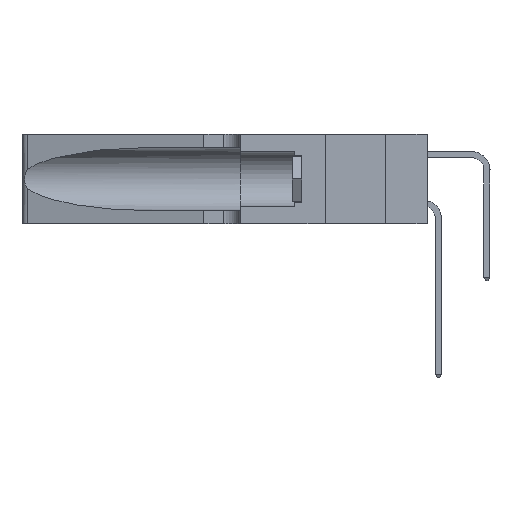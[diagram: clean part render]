
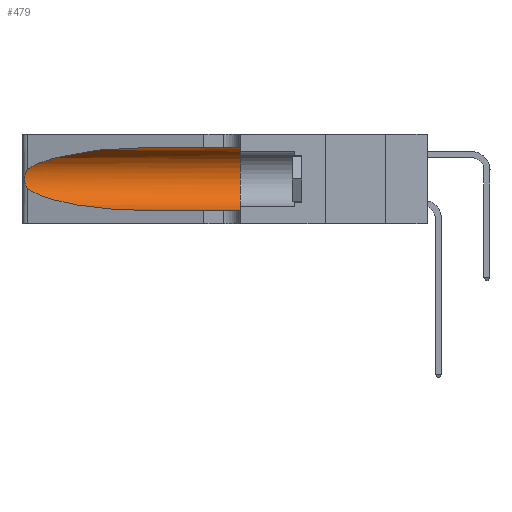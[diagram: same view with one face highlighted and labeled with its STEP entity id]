
A CAD part, left-side view. The second image highlights one B-rep face of the part: STEP entity #479.
In plain terms, the highlighted cylindrical face has radius 3.308 mm (diameter 6.617 mm), a partial arc.
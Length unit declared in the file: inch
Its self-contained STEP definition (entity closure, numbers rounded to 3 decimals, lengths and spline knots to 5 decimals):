
#324 = EDGE_CURVE ( 'NONE', #16394, #5840, #4225, .T. ) ;
#479 = ADVANCED_FACE ( 'NONE', ( #18718 ), #23139, .F. ) ;
#1577 = ORIENTED_EDGE ( 'NONE', *, *, #3728, .T. ) ;
#1714 = CARTESIAN_POINT ( 'NONE',  ( 0.1305, 0.35, 0.31525 ) ) ;
#1887 = CARTESIAN_POINT ( 'NONE',  ( 0.25639, 1.23186, 0.15144 ) ) ;
#2114 = EDGE_LOOP ( 'NONE', ( #1577, #14089, #24258, #11299, #9161, #21161 ) ) ;
#3728 = EDGE_CURVE ( 'NONE', #9143, #12428, #3777, .T. ) ;
#3777 =( BOUNDED_CURVE ( )  B_SPLINE_CURVE ( 3, ( #7094, #5178, #16529, #20314 ),
 .UNSPECIFIED., .F., .T. ) 
 B_SPLINE_CURVE_WITH_KNOTS ( ( 4, 4 ),
 ( 1.5708, 2.84003 ),
 .UNSPECIFIED. ) 
 CURVE ( )  GEOMETRIC_REPRESENTATION_ITEM ( )  RATIONAL_B_SPLINE_CURVE ( ( 1., 0.87, 0.87, 1. ) ) 
 REPRESENTATION_ITEM ( '' )  );
#3819 = CARTESIAN_POINT ( 'NONE',  ( 0.25487, 1.22718, 0.14631 ) ) ;
#4225 =( BOUNDED_CURVE ( )  B_SPLINE_CURVE ( 3, ( #23592, #22608, #22773, #18902 ),
 .UNSPECIFIED., .F., .T. ) 
 B_SPLINE_CURVE_WITH_KNOTS ( ( 4, 4 ),
 ( 3.44316, 4.71239 ),
 .UNSPECIFIED. ) 
 CURVE ( )  GEOMETRIC_REPRESENTATION_ITEM ( )  RATIONAL_B_SPLINE_CURVE ( ( 1., 0.87, 0.87, 1. ) ) 
 REPRESENTATION_ITEM ( '' )  );
#4977 = EDGE_CURVE ( 'NONE', #21585, #9734, #11578, .T. ) ;
#5178 = CARTESIAN_POINT ( 'NONE',  ( 0.18966, 0.96281, 0.31525 ) ) ;
#5443 = LINE ( 'NONE', #18367, #14940 ) ;
#5587 = CARTESIAN_POINT ( 'NONE',  ( 0.25487, 1.22718, 0.22369 ) ) ;
#5673 = CARTESIAN_POINT ( 'NONE',  ( 0.25639, 1.23184, 0.21858 ) ) ;
#5686 = CARTESIAN_POINT ( 'NONE',  ( 0.1305, 0.72297, 0.05475 ) ) ;
#5840 = VERTEX_POINT ( 'NONE', #5686 ) ;
#6756 = CARTESIAN_POINT ( 'NONE',  ( 0.1305, 0.72297, 0.31525 ) ) ;
#7094 = CARTESIAN_POINT ( 'NONE',  ( 0.1305, 0.72297, 0.31525 ) ) ;
#7126 = DIRECTION ( 'NONE',  ( 0., 1., 0. ) ) ;
#7581 = CARTESIAN_POINT ( 'NONE',  ( 0.25854, 1.2359, 0.20912 ) ) ;
#8857 = DIRECTION ( 'NONE',  ( 0., 0., -1. ) ) ;
#8878 = CARTESIAN_POINT ( 'NONE',  ( 0.1305, 0.35, 0.05475 ) ) ;
#9143 = VERTEX_POINT ( 'NONE', #6756 ) ;
#9161 = ORIENTED_EDGE ( 'NONE', *, *, #4977, .F. ) ;
#9429 = CARTESIAN_POINT ( 'NONE',  ( 0.1305, 1.61858, 0.185 ) ) ;
#9481 = CARTESIAN_POINT ( 'NONE',  ( 0.26075, 1.23896, 0.19203 ) ) ;
#9734 = VERTEX_POINT ( 'NONE', #8878 ) ;
#10153 = AXIS2_PLACEMENT_3D ( 'NONE', #9429, #11488, #8857 ) ;
#11299 = ORIENTED_EDGE ( 'NONE', *, *, #22690, .T. ) ;
#11385 = CARTESIAN_POINT ( 'NONE',  ( 0.26017, 1.23833, 0.17102 ) ) ;
#11488 = DIRECTION ( 'NONE',  ( 0., -1., 0. ) ) ;
#11578 = CIRCLE ( 'NONE', #17966, 0.13025 ) ;
#12428 = VERTEX_POINT ( 'NONE', #16102 ) ;
#13272 = CARTESIAN_POINT ( 'NONE',  ( 0.25789, 1.23486, 0.15765 ) ) ;
#13274 = CARTESIAN_POINT ( 'NONE',  ( 0.25487, 1.22718, 0.14631 ) ) ;
#14089 = ORIENTED_EDGE ( 'NONE', *, *, #24045, .T. ) ;
#14370 = LINE ( 'NONE', #21673, #23793 ) ;
#14940 = VECTOR ( 'NONE', #24059, 39.37008 ) ;
#15016 = EDGE_CURVE ( 'NONE', #9143, #21585, #14370, .T. ) ;
#15114 = CARTESIAN_POINT ( 'NONE',  ( 0.25555, 1.22994, 0.2215 ) ) ;
#15202 = CARTESIAN_POINT ( 'NONE',  ( 0.25555, 1.22993, 0.14849 ) ) ;
#16102 = CARTESIAN_POINT ( 'NONE',  ( 0.25487, 1.22718, 0.22369 ) ) ;
#16394 = VERTEX_POINT ( 'NONE', #13274 ) ;
#16529 = CARTESIAN_POINT ( 'NONE',  ( 0.2373, 1.15595, 0.28018 ) ) ;
#17892 = DIRECTION ( 'NONE',  ( 0., -1., 0. ) ) ;
#17966 = AXIS2_PLACEMENT_3D ( 'NONE', #18440, #7126, #20348 ) ;
#18367 = CARTESIAN_POINT ( 'NONE',  ( 0.1305, 1.61858, 0.05475 ) ) ;
#18440 = CARTESIAN_POINT ( 'NONE',  ( 0.1305, 0.35, 0.185 ) ) ;
#18718 = FACE_OUTER_BOUND ( 'NONE', #2114, .T. ) ;
#18900 = CARTESIAN_POINT ( 'NONE',  ( 0.25787, 1.23484, 0.2124 ) ) ;
#18902 = CARTESIAN_POINT ( 'NONE',  ( 0.1305, 0.72297, 0.05475 ) ) ;
#20314 = CARTESIAN_POINT ( 'NONE',  ( 0.25487, 1.22718, 0.22369 ) ) ;
#20348 = DIRECTION ( 'NONE',  ( 0., 0., 1. ) ) ;
#20794 = CARTESIAN_POINT ( 'NONE',  ( 0.26018, 1.23835, 0.19895 ) ) ;
#21161 = ORIENTED_EDGE ( 'NONE', *, *, #15016, .F. ) ;
#21368 = CARTESIAN_POINT ( 'NONE',  ( 0.25856, 1.23593, 0.16098 ) ) ;
#21585 = VERTEX_POINT ( 'NONE', #1714 ) ;
#21673 = CARTESIAN_POINT ( 'NONE',  ( 0.1305, 1.61858, 0.31525 ) ) ;
#22608 = CARTESIAN_POINT ( 'NONE',  ( 0.2373, 1.15595, 0.08982 ) ) ;
#22686 = CARTESIAN_POINT ( 'NONE',  ( 0.26075, 1.23896, 0.178 ) ) ;
#22690 = EDGE_CURVE ( 'NONE', #5840, #9734, #5443, .T. ) ;
#22773 = CARTESIAN_POINT ( 'NONE',  ( 0.18966, 0.96281, 0.05475 ) ) ;
#23139 = CYLINDRICAL_SURFACE ( 'NONE', #10153, 0.13025 ) ;
#23592 = CARTESIAN_POINT ( 'NONE',  ( 0.25487, 1.22718, 0.14631 ) ) ;
#23793 = VECTOR ( 'NONE', #17892, 39.37008 ) ;
#24045 = EDGE_CURVE ( 'NONE', #12428, #16394, #24094, .T. ) ;
#24059 = DIRECTION ( 'NONE',  ( 0., -1., 0. ) ) ;
#24094 = B_SPLINE_CURVE_WITH_KNOTS ( 'NONE', 3,
 ( #5587, #15114, #5673, #18900, #7581, #20794, #9481, #22686, #11385, #21368, #13272, #1887, #15202, #3819 ),
 .UNSPECIFIED., .F., .F.,
 ( 4, 2, 2, 2, 2, 2, 4 ),
 ( 0., 0.00027, 0.00053, 0.00107, 0.0016, 0.00187, 0.00214 ),
 .UNSPECIFIED. ) ;
#24258 = ORIENTED_EDGE ( 'NONE', *, *, #324, .T. ) ;
